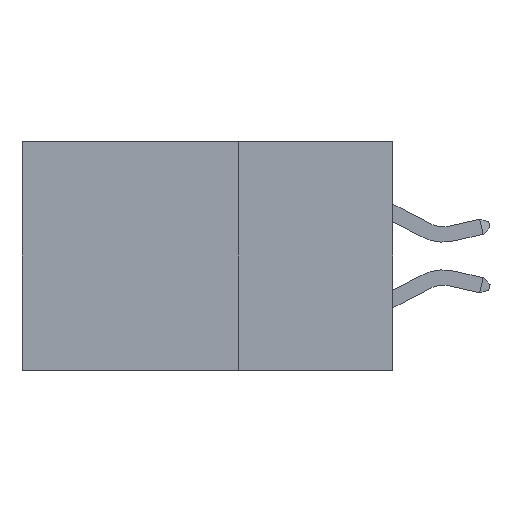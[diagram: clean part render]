
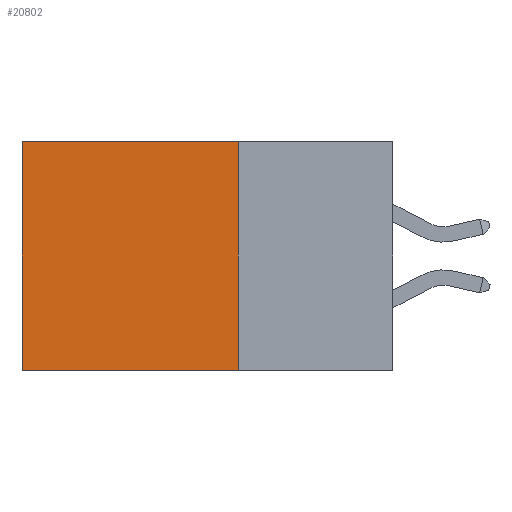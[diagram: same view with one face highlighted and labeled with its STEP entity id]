
A CAD part, left-side view. The second image highlights one B-rep face of the part: STEP entity #20802.
In plain terms, the highlighted planar face has unit normal (-1, 0, 0).
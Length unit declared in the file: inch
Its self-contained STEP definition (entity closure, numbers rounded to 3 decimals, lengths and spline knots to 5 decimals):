
#167 = VERTEX_POINT ( 'NONE', #2030 ) ;
#502 = CARTESIAN_POINT ( 'NONE',  ( 0.2875, 0.6, 0. ) ) ;
#1460 = VECTOR ( 'NONE', #14391, 39.37008 ) ;
#2030 = CARTESIAN_POINT ( 'NONE',  ( 0.2875, 0.6, -0.37 ) ) ;
#3055 = ORIENTED_EDGE ( 'NONE', *, *, #10875, .T. ) ;
#3517 = ORIENTED_EDGE ( 'NONE', *, *, #21421, .F. ) ;
#3655 = EDGE_CURVE ( 'NONE', #7698, #19272, #6174, .T. ) ;
#3919 = CARTESIAN_POINT ( 'NONE',  ( 0.2875, 0.25, 0. ) ) ;
#4106 = EDGE_CURVE ( 'NONE', #7698, #8728, #15231, .T. ) ;
#4503 = DIRECTION ( 'NONE',  ( 0., 1., 0. ) ) ;
#6174 = LINE ( 'NONE', #9893, #10698 ) ;
#6379 = VECTOR ( 'NONE', #4503, 39.37008 ) ;
#6518 = CARTESIAN_POINT ( 'NONE',  ( 0.2875, 0.25, 0. ) ) ;
#6713 = ORIENTED_EDGE ( 'NONE', *, *, #3655, .T. ) ;
#7698 = VERTEX_POINT ( 'NONE', #3919 ) ;
#8728 = VERTEX_POINT ( 'NONE', #15071 ) ;
#9893 = CARTESIAN_POINT ( 'NONE',  ( 0.2875, 0.25, 0. ) ) ;
#10567 = ORIENTED_EDGE ( 'NONE', *, *, #4106, .F. ) ;
#10573 = AXIS2_PLACEMENT_3D ( 'NONE', #6518, #21774, #11630 ) ;
#10674 = VECTOR ( 'NONE', #11106, 39.37008 ) ;
#10698 = VECTOR ( 'NONE', #11580, 39.37008 ) ;
#10875 = EDGE_CURVE ( 'NONE', #19272, #167, #15101, .T. ) ;
#11106 = DIRECTION ( 'NONE',  ( 0., 0., -1. ) ) ;
#11412 = LINE ( 'NONE', #16431, #6379 ) ;
#11580 = DIRECTION ( 'NONE',  ( 0., 1., 0. ) ) ;
#11630 = DIRECTION ( 'NONE',  ( 0., 0., -1. ) ) ;
#12654 = CARTESIAN_POINT ( 'NONE',  ( 0.2875, 0.6, 0. ) ) ;
#14391 = DIRECTION ( 'NONE',  ( 0., 0., -1. ) ) ;
#14904 = FACE_OUTER_BOUND ( 'NONE', #16898, .T. ) ;
#15020 = PLANE ( 'NONE',  #10573 ) ;
#15071 = CARTESIAN_POINT ( 'NONE',  ( 0.2875, 0.25, -0.37 ) ) ;
#15101 = LINE ( 'NONE', #12654, #1460 ) ;
#15231 = LINE ( 'NONE', #21278, #10674 ) ;
#16431 = CARTESIAN_POINT ( 'NONE',  ( 0.2875, 0.25, -0.37 ) ) ;
#16898 = EDGE_LOOP ( 'NONE', ( #3055, #3517, #10567, #6713 ) ) ;
#19272 = VERTEX_POINT ( 'NONE', #502 ) ;
#20802 = ADVANCED_FACE ( 'NONE', ( #14904 ), #15020, .F. ) ;
#21278 = CARTESIAN_POINT ( 'NONE',  ( 0.2875, 0.25, 0. ) ) ;
#21421 = EDGE_CURVE ( 'NONE', #8728, #167, #11412, .T. ) ;
#21774 = DIRECTION ( 'NONE',  ( 1., 0., 0. ) ) ;
